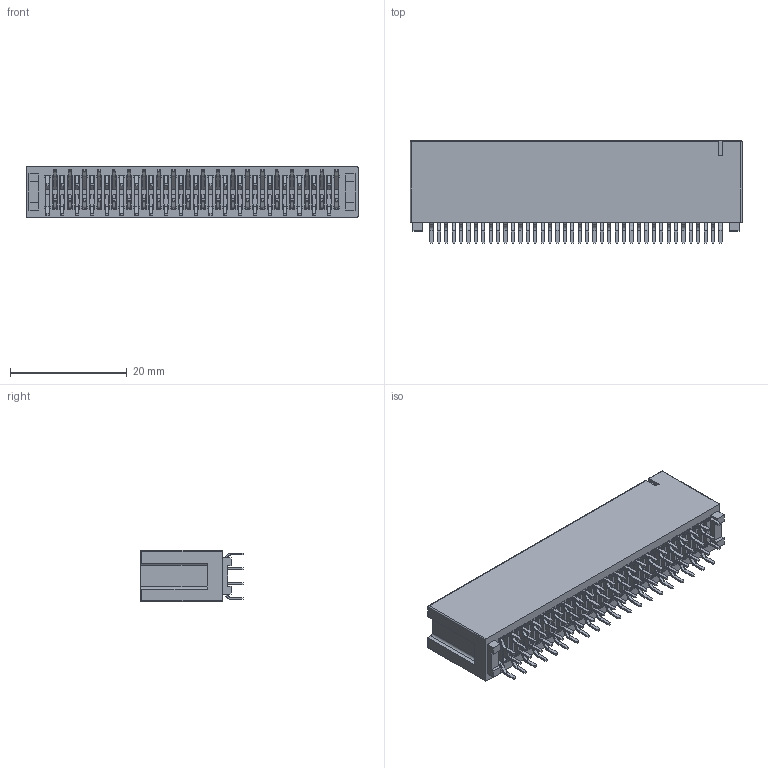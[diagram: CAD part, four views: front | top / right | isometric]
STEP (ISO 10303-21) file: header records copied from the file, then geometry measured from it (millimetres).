
FILE_DESCRIPTION (( 'STEP AP203' ), '1' );
FILE_NAME ('302-080-321-201.STEP', '2024-04-01T19:34:00', ( '' ), ( '' ), 'SwSTEP 2.0', 'SolidWorks 2023', '' );
FILE_SCHEMA (( 'CONFIG_CONTROL_DESIGN' ));
Length unit declared in the file: millimetre
Products named in the file (4): HSG_Vertical HSG; Contact_302-290-X21 (2); 302-080-321-201; Contact_302-290-X21 (1)
Assembly tree (81 placements, depth 2):
  302-080-321-201
    HSG_Vertical HSG
    Contact_302-290-X21 (2)  x40
    Contact_302-290-X21 (1)  x40
Bounding box: 56.9 x 17.63 x 8.88 mm (x, y, z)
Volume: 4394.3 mm3; surface area: 12188.4 mm2
Topology: 81 solids, 81 shells, 3706 faces, 10888 edges, 7144 vertices
Faces by surface type: plane 2729, cylinder 813, bspline 160, sphere 4
Entity records: 32336 total; most frequent: ORIENTED_EDGE 5544, CARTESIAN_POINT 5542, DIRECTION 4474, EDGE_CURVE 2772, LINE 2698, VECTOR 2698, VERTEX_POINT 1840, AXIS2_PLACEMENT_3D 888
